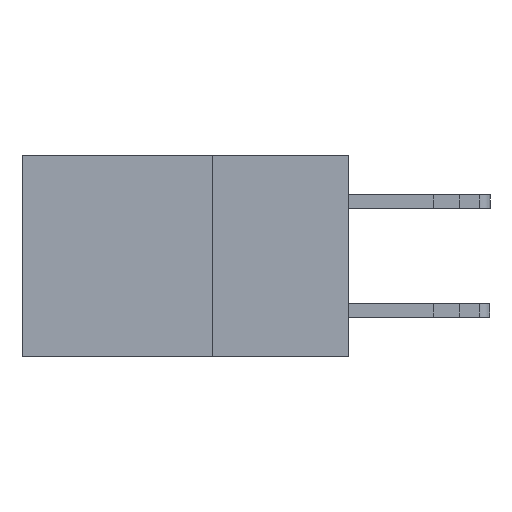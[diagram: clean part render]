
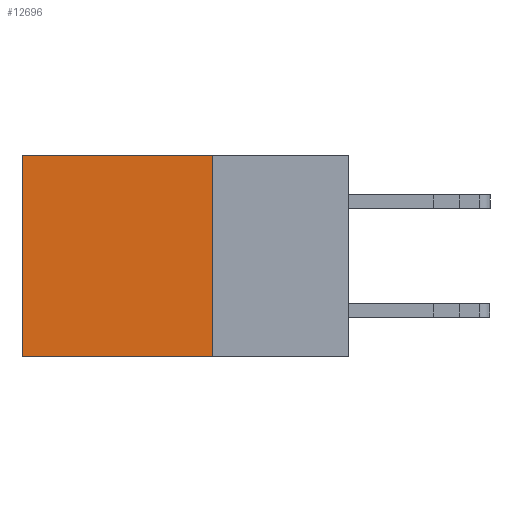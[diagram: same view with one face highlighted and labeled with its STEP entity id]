
A CAD part, left-side view. The second image highlights one B-rep face of the part: STEP entity #12696.
In plain terms, the highlighted planar face has unit normal (-1, 0, 0).
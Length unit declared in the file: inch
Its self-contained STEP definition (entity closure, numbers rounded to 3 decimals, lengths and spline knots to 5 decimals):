
#504 = EDGE_CURVE ( 'NONE', #20852, #3173, #2413, .T. ) ;
#982 = EDGE_LOOP ( 'NONE', ( #5527, #10257, #10232, #21664 ) ) ;
#2413 = LINE ( 'NONE', #13374, #11069 ) ;
#3173 = VERTEX_POINT ( 'NONE', #20807 ) ;
#3249 = EDGE_CURVE ( 'NONE', #3832, #20852, #3663, .T. ) ;
#3349 = LINE ( 'NONE', #9507, #9528 ) ;
#3663 = LINE ( 'NONE', #6711, #21315 ) ;
#3832 = VERTEX_POINT ( 'NONE', #12324 ) ;
#4068 = CARTESIAN_POINT ( 'NONE',  ( 0.298, 0.25, -0.37 ) ) ;
#4353 = DIRECTION ( 'NONE',  ( 0., 1., 0. ) ) ;
#5527 = ORIENTED_EDGE ( 'NONE', *, *, #504, .T. ) ;
#5714 = DIRECTION ( 'NONE',  ( 0., 1., 0. ) ) ;
#6455 = AXIS2_PLACEMENT_3D ( 'NONE', #8932, #19330, #9010 ) ;
#6711 = CARTESIAN_POINT ( 'NONE',  ( 0.298, 0.25, 0. ) ) ;
#8023 = VECTOR ( 'NONE', #4353, 39.37008 ) ;
#8932 = CARTESIAN_POINT ( 'NONE',  ( 0.298, 0.25, 0. ) ) ;
#9010 = DIRECTION ( 'NONE',  ( 0., 0., -1. ) ) ;
#9507 = CARTESIAN_POINT ( 'NONE',  ( 0.298, 0.25, 0. ) ) ;
#9528 = VECTOR ( 'NONE', #11257, 39.37008 ) ;
#9607 = EDGE_CURVE ( 'NONE', #12774, #3173, #21641, .T. ) ;
#10232 = ORIENTED_EDGE ( 'NONE', *, *, #19435, .F. ) ;
#10257 = ORIENTED_EDGE ( 'NONE', *, *, #9607, .F. ) ;
#11069 = VECTOR ( 'NONE', #13405, 39.37008 ) ;
#11257 = DIRECTION ( 'NONE',  ( 0., 0., -1. ) ) ;
#12324 = CARTESIAN_POINT ( 'NONE',  ( 0.298, 0.25, 0. ) ) ;
#12696 = ADVANCED_FACE ( 'NONE', ( #16165 ), #17631, .F. ) ;
#12774 = VERTEX_POINT ( 'NONE', #4068 ) ;
#13374 = CARTESIAN_POINT ( 'NONE',  ( 0.298, 0.6, 0. ) ) ;
#13405 = DIRECTION ( 'NONE',  ( 0., 0., -1. ) ) ;
#16165 = FACE_OUTER_BOUND ( 'NONE', #982, .T. ) ;
#17631 = PLANE ( 'NONE',  #6455 ) ;
#19330 = DIRECTION ( 'NONE',  ( 1., 0., 0. ) ) ;
#19435 = EDGE_CURVE ( 'NONE', #3832, #12774, #3349, .T. ) ;
#19745 = CARTESIAN_POINT ( 'NONE',  ( 0.298, 0.25, -0.37 ) ) ;
#20723 = CARTESIAN_POINT ( 'NONE',  ( 0.298, 0.6, 0. ) ) ;
#20807 = CARTESIAN_POINT ( 'NONE',  ( 0.298, 0.6, -0.37 ) ) ;
#20852 = VERTEX_POINT ( 'NONE', #20723 ) ;
#21315 = VECTOR ( 'NONE', #5714, 39.37008 ) ;
#21641 = LINE ( 'NONE', #19745, #8023 ) ;
#21664 = ORIENTED_EDGE ( 'NONE', *, *, #3249, .T. ) ;
